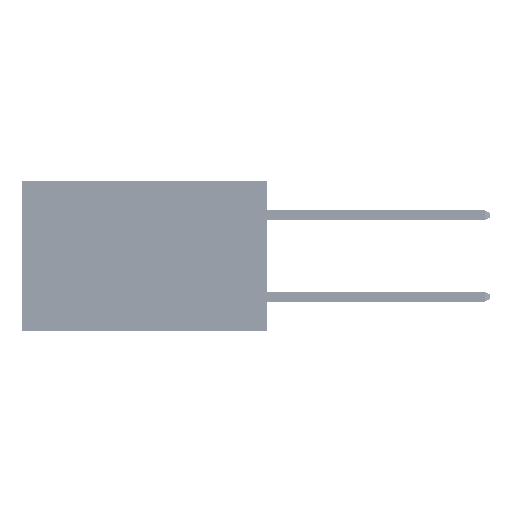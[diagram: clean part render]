
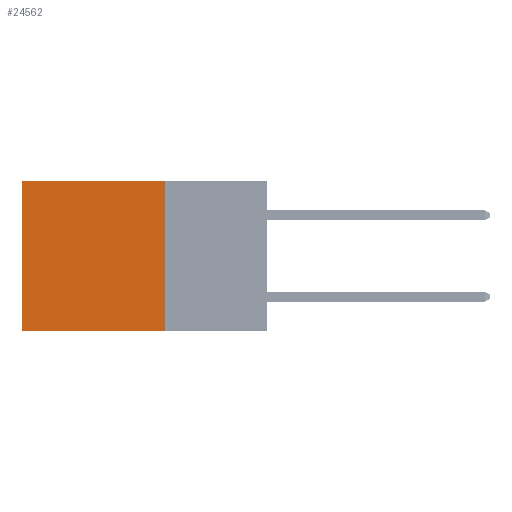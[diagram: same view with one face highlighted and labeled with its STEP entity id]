
A CAD part, left-side view. The second image highlights one B-rep face of the part: STEP entity #24562.
In plain terms, the highlighted planar face has unit normal (-1, 0, 0).
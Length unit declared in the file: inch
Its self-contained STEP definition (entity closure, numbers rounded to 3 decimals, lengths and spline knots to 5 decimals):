
#270 = DIRECTION ( 'NONE',  ( 0., 0., -1. ) ) ;
#1612 = VERTEX_POINT ( 'NONE', #44326 ) ;
#2149 = LINE ( 'NONE', #46626, #12420 ) ;
#3418 = VECTOR ( 'NONE', #27444, 39.37008 ) ;
#5546 = EDGE_CURVE ( 'NONE', #23608, #1612, #46585, .T. ) ;
#6092 = DIRECTION ( 'NONE',  ( 0., 0., -1. ) ) ;
#10080 = CARTESIAN_POINT ( 'NONE',  ( 0.2875, 0.25, 0. ) ) ;
#12230 = VERTEX_POINT ( 'NONE', #32125 ) ;
#12420 = VECTOR ( 'NONE', #38404, 39.37008 ) ;
#12901 = ORIENTED_EDGE ( 'NONE', *, *, #5546, .F. ) ;
#15409 = CARTESIAN_POINT ( 'NONE',  ( 0.2875, 0.25, 0. ) ) ;
#21829 = ORIENTED_EDGE ( 'NONE', *, *, #27975, .T. ) ;
#22167 = EDGE_CURVE ( 'NONE', #1612, #12230, #2149, .T. ) ;
#23491 = DIRECTION ( 'NONE',  ( 1., 0., 0. ) ) ;
#23608 = VERTEX_POINT ( 'NONE', #15409 ) ;
#23661 = ORIENTED_EDGE ( 'NONE', *, *, #25942, .T. ) ;
#24562 = ADVANCED_FACE ( 'NONE', ( #40127 ), #43847, .F. ) ;
#25942 = EDGE_CURVE ( 'NONE', #51633, #12230, #49737, .T. ) ;
#27444 = DIRECTION ( 'NONE',  ( 0., 1., 0. ) ) ;
#27975 = EDGE_CURVE ( 'NONE', #23608, #51633, #35364, .T. ) ;
#28249 = DIRECTION ( 'NONE',  ( 0., 0., -1. ) ) ;
#28862 = CARTESIAN_POINT ( 'NONE',  ( 0.2875, 0.6, 0. ) ) ;
#32125 = CARTESIAN_POINT ( 'NONE',  ( 0.2875, 0.6, -0.37 ) ) ;
#35364 = LINE ( 'NONE', #40115, #3418 ) ;
#35892 = CARTESIAN_POINT ( 'NONE',  ( 0.2875, 0.25, 0. ) ) ;
#37038 = VECTOR ( 'NONE', #6092, 39.37008 ) ;
#38404 = DIRECTION ( 'NONE',  ( 0., 1., 0. ) ) ;
#40115 = CARTESIAN_POINT ( 'NONE',  ( 0.2875, 0.25, 0. ) ) ;
#40127 = FACE_OUTER_BOUND ( 'NONE', #44239, .T. ) ;
#42118 = VECTOR ( 'NONE', #270, 39.37008 ) ;
#43847 = PLANE ( 'NONE',  #52187 ) ;
#44239 = EDGE_LOOP ( 'NONE', ( #23661, #50809, #12901, #21829 ) ) ;
#44326 = CARTESIAN_POINT ( 'NONE',  ( 0.2875, 0.25, -0.37 ) ) ;
#46585 = LINE ( 'NONE', #10080, #37038 ) ;
#46626 = CARTESIAN_POINT ( 'NONE',  ( 0.2875, 0.25, -0.37 ) ) ;
#49737 = LINE ( 'NONE', #28862, #42118 ) ;
#50809 = ORIENTED_EDGE ( 'NONE', *, *, #22167, .F. ) ;
#51633 = VERTEX_POINT ( 'NONE', #52070 ) ;
#52070 = CARTESIAN_POINT ( 'NONE',  ( 0.2875, 0.6, 0. ) ) ;
#52187 = AXIS2_PLACEMENT_3D ( 'NONE', #35892, #23491, #28249 ) ;
